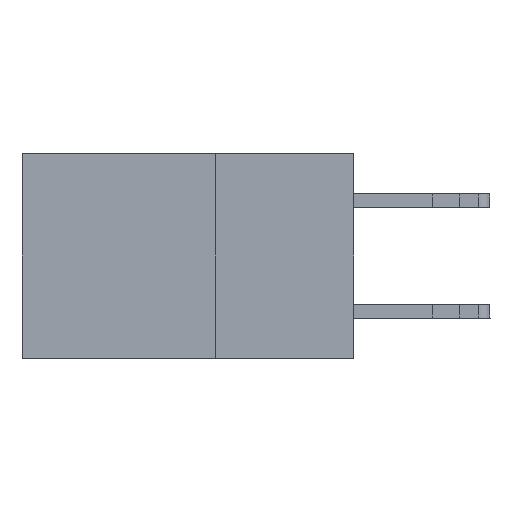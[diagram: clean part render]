
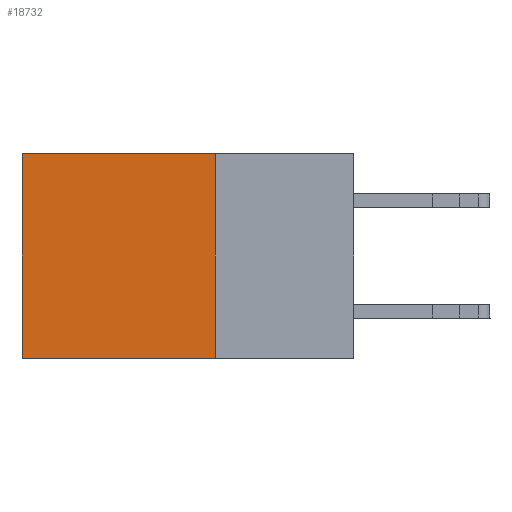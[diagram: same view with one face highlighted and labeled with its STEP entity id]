
A CAD part, left-side view. The second image highlights one B-rep face of the part: STEP entity #18732.
In plain terms, the highlighted planar face has unit normal (-1, 0, 0).
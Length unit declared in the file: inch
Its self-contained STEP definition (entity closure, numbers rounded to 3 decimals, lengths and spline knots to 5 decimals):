
#621 = EDGE_CURVE ( 'NONE', #21327, #16373, #6855, .T. ) ;
#3760 = DIRECTION ( 'NONE',  ( 0., 0., -1. ) ) ;
#5579 = LINE ( 'NONE', #20648, #15631 ) ;
#6855 = LINE ( 'NONE', #14386, #13465 ) ;
#7708 = VERTEX_POINT ( 'NONE', #22251 ) ;
#8019 = CARTESIAN_POINT ( 'NONE',  ( 0.2875, 0.25, -0.37 ) ) ;
#8576 = CARTESIAN_POINT ( 'NONE',  ( 0.2875, 0.25, 0. ) ) ;
#9234 = EDGE_CURVE ( 'NONE', #16373, #7708, #17174, .T. ) ;
#9282 = CARTESIAN_POINT ( 'NONE',  ( 0.2875, 0.6, 0. ) ) ;
#9371 = DIRECTION ( 'NONE',  ( 0., 1., 0. ) ) ;
#10633 = ORIENTED_EDGE ( 'NONE', *, *, #19107, .F. ) ;
#11123 = CARTESIAN_POINT ( 'NONE',  ( 0.2875, 0.25, -0.37 ) ) ;
#11977 = AXIS2_PLACEMENT_3D ( 'NONE', #8576, #12525, #17870 ) ;
#12010 = CARTESIAN_POINT ( 'NONE',  ( 0.2875, 0.25, 0. ) ) ;
#12525 = DIRECTION ( 'NONE',  ( 1., 0., 0. ) ) ;
#13324 = LINE ( 'NONE', #8019, #14249 ) ;
#13465 = VECTOR ( 'NONE', #24006, 39.37008 ) ;
#14249 = VECTOR ( 'NONE', #9371, 39.37008 ) ;
#14278 = PLANE ( 'NONE',  #11977 ) ;
#14386 = CARTESIAN_POINT ( 'NONE',  ( 0.2875, 0.25, 0. ) ) ;
#14984 = EDGE_CURVE ( 'NONE', #21327, #22903, #5579, .T. ) ;
#15335 = EDGE_LOOP ( 'NONE', ( #18940, #10633, #21720, #19239 ) ) ;
#15631 = VECTOR ( 'NONE', #3760, 39.37008 ) ;
#16373 = VERTEX_POINT ( 'NONE', #9282 ) ;
#17174 = LINE ( 'NONE', #22823, #21743 ) ;
#17870 = DIRECTION ( 'NONE',  ( 0., 0., -1. ) ) ;
#18732 = ADVANCED_FACE ( 'NONE', ( #22049 ), #14278, .F. ) ;
#18940 = ORIENTED_EDGE ( 'NONE', *, *, #9234, .T. ) ;
#19107 = EDGE_CURVE ( 'NONE', #22903, #7708, #13324, .T. ) ;
#19149 = DIRECTION ( 'NONE',  ( 0., 0., -1. ) ) ;
#19239 = ORIENTED_EDGE ( 'NONE', *, *, #621, .T. ) ;
#20648 = CARTESIAN_POINT ( 'NONE',  ( 0.2875, 0.25, 0. ) ) ;
#21327 = VERTEX_POINT ( 'NONE', #12010 ) ;
#21720 = ORIENTED_EDGE ( 'NONE', *, *, #14984, .F. ) ;
#21743 = VECTOR ( 'NONE', #19149, 39.37008 ) ;
#22049 = FACE_OUTER_BOUND ( 'NONE', #15335, .T. ) ;
#22251 = CARTESIAN_POINT ( 'NONE',  ( 0.2875, 0.6, -0.37 ) ) ;
#22823 = CARTESIAN_POINT ( 'NONE',  ( 0.2875, 0.6, 0. ) ) ;
#22903 = VERTEX_POINT ( 'NONE', #11123 ) ;
#24006 = DIRECTION ( 'NONE',  ( 0., 1., 0. ) ) ;
